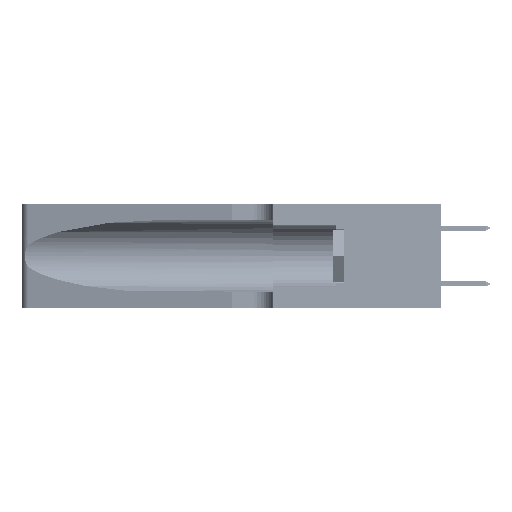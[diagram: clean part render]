
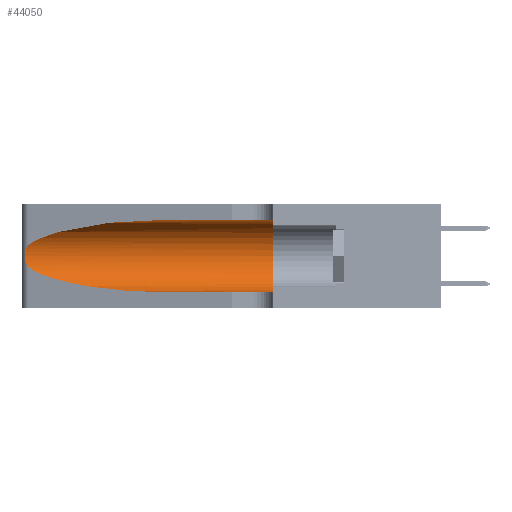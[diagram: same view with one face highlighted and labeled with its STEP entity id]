
A CAD part, left-side view. The second image highlights one B-rep face of the part: STEP entity #44050.
In plain terms, the highlighted cylindrical face has radius 3.308 mm (diameter 6.617 mm), a partial arc.
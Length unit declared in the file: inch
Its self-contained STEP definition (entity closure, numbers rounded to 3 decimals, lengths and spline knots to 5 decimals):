
#435 = EDGE_CURVE ( 'NONE', #28097, #11535, #31660, .T. ) ;
#770 =( BOUNDED_CURVE ( )  B_SPLINE_CURVE ( 3, ( #2376, #9634, #16891, #41782 ),
 .UNSPECIFIED., .F., .F. ) 
 B_SPLINE_CURVE_WITH_KNOTS ( ( 4, 4 ),
 ( 1.5708, 2.84003 ),
 .UNSPECIFIED. ) 
 CURVE ( )  GEOMETRIC_REPRESENTATION_ITEM ( )  RATIONAL_B_SPLINE_CURVE ( ( 1., 0.87, 0.87, 1. ) ) 
 REPRESENTATION_ITEM ( '' )  );
#802 = DIRECTION ( 'NONE',  ( 0., 0., -1. ) ) ;
#2350 = CARTESIAN_POINT ( 'NONE',  ( 0.1305, 0.72297, 0.05475 ) ) ;
#2376 = CARTESIAN_POINT ( 'NONE',  ( 0.1305, 0.72297, 0.31525 ) ) ;
#3324 = ORIENTED_EDGE ( 'NONE', *, *, #16526, .F. ) ;
#3594 = CARTESIAN_POINT ( 'NONE',  ( 0.25639, 1.23186, 0.15144 ) ) ;
#6356 = CIRCLE ( 'NONE', #20125, 0.13025 ) ;
#7041 = CARTESIAN_POINT ( 'NONE',  ( 0.25555, 1.22994, 0.2215 ) ) ;
#7211 = CARTESIAN_POINT ( 'NONE',  ( 0.25487, 1.22718, 0.14631 ) ) ;
#7308 = EDGE_CURVE ( 'NONE', #9059, #24847, #37540, .T. ) ;
#8315 = CARTESIAN_POINT ( 'NONE',  ( 0.1305, 1.61858, 0.31525 ) ) ;
#8981 = VECTOR ( 'NONE', #22876, 39.37008 ) ;
#9059 = VERTEX_POINT ( 'NONE', #37400 ) ;
#9634 = CARTESIAN_POINT ( 'NONE',  ( 0.18966, 0.96281, 0.31525 ) ) ;
#10125 = AXIS2_PLACEMENT_3D ( 'NONE', #22480, #15165, #802 ) ;
#10717 = CARTESIAN_POINT ( 'NONE',  ( 0.25639, 1.23184, 0.21858 ) ) ;
#10972 = CARTESIAN_POINT ( 'NONE',  ( 0.2373, 1.15595, 0.08982 ) ) ;
#11535 = VERTEX_POINT ( 'NONE', #2350 ) ;
#13559 = CARTESIAN_POINT ( 'NONE',  ( 0.25487, 1.22718, 0.22369 ) ) ;
#13665 = EDGE_CURVE ( 'NONE', #30911, #28097, #21604, .T. ) ;
#14311 = CARTESIAN_POINT ( 'NONE',  ( 0.25854, 1.2359, 0.20912 ) ) ;
#15165 = DIRECTION ( 'NONE',  ( 0., -1., 0. ) ) ;
#15543 = CARTESIAN_POINT ( 'NONE',  ( 0.25487, 1.22718, 0.14631 ) ) ;
#16480 = CARTESIAN_POINT ( 'NONE',  ( 0.1305, 1.61858, 0.05475 ) ) ;
#16526 = EDGE_CURVE ( 'NONE', #24847, #32883, #6356, .T. ) ;
#16591 = CARTESIAN_POINT ( 'NONE',  ( 0.1305, 0.35, 0.31525 ) ) ;
#16891 = CARTESIAN_POINT ( 'NONE',  ( 0.2373, 1.15595, 0.28018 ) ) ;
#17970 = CARTESIAN_POINT ( 'NONE',  ( 0.26075, 1.23896, 0.19203 ) ) ;
#18861 = EDGE_CURVE ( 'NONE', #9059, #30911, #770, .T. ) ;
#19762 = CARTESIAN_POINT ( 'NONE',  ( 0.25856, 1.23593, 0.16098 ) ) ;
#19768 = DIRECTION ( 'NONE',  ( 0., 1., 0. ) ) ;
#20125 = AXIS2_PLACEMENT_3D ( 'NONE', #41024, #19768, #44546 ) ;
#20153 = DIRECTION ( 'NONE',  ( 0., -1., 0. ) ) ;
#20657 = VECTOR ( 'NONE', #20153, 39.37008 ) ;
#21604 = B_SPLINE_CURVE_WITH_KNOTS ( 'NONE', 3,
 ( #39135, #7041, #10717, #35744, #14311, #39286, #17970, #42828, #21638, #19762, #25254, #3594, #28826, #7211 ),
 .UNSPECIFIED., .F., .F.,
 ( 4, 2, 2, 2, 2, 2, 4 ),
 ( 0., 0.00027, 0.00053, 0.00107, 0.0016, 0.00187, 0.00214 ),
 .UNSPECIFIED. ) ;
#21638 = CARTESIAN_POINT ( 'NONE',  ( 0.26017, 1.23833, 0.17102 ) ) ;
#21849 = CARTESIAN_POINT ( 'NONE',  ( 0.1305, 0.35, 0.05475 ) ) ;
#21883 = EDGE_CURVE ( 'NONE', #11535, #32883, #38412, .T. ) ;
#22182 = CYLINDRICAL_SURFACE ( 'NONE', #10125, 0.13025 ) ;
#22480 = CARTESIAN_POINT ( 'NONE',  ( 0.1305, 1.61858, 0.185 ) ) ;
#22876 = DIRECTION ( 'NONE',  ( 0., -1., 0. ) ) ;
#24847 = VERTEX_POINT ( 'NONE', #16591 ) ;
#25254 = CARTESIAN_POINT ( 'NONE',  ( 0.25789, 1.23486, 0.15765 ) ) ;
#25903 = ORIENTED_EDGE ( 'NONE', *, *, #18861, .T. ) ;
#27582 = ORIENTED_EDGE ( 'NONE', *, *, #21883, .T. ) ;
#28097 = VERTEX_POINT ( 'NONE', #15543 ) ;
#28826 = CARTESIAN_POINT ( 'NONE',  ( 0.25555, 1.22993, 0.14849 ) ) ;
#30911 = VERTEX_POINT ( 'NONE', #13559 ) ;
#31660 =( BOUNDED_CURVE ( )  B_SPLINE_CURVE ( 3, ( #35997, #10972, #32488, #39542 ),
 .UNSPECIFIED., .F., .F. ) 
 B_SPLINE_CURVE_WITH_KNOTS ( ( 4, 4 ),
 ( 3.44316, 4.71239 ),
 .UNSPECIFIED. ) 
 CURVE ( )  GEOMETRIC_REPRESENTATION_ITEM ( )  RATIONAL_B_SPLINE_CURVE ( ( 1., 0.87, 0.87, 1. ) ) 
 REPRESENTATION_ITEM ( '' )  );
#32488 = CARTESIAN_POINT ( 'NONE',  ( 0.18966, 0.96281, 0.05475 ) ) ;
#32883 = VERTEX_POINT ( 'NONE', #21849 ) ;
#32924 = EDGE_LOOP ( 'NONE', ( #25903, #43014, #35848, #27582, #3324, #34243 ) ) ;
#34243 = ORIENTED_EDGE ( 'NONE', *, *, #7308, .F. ) ;
#35744 = CARTESIAN_POINT ( 'NONE',  ( 0.25787, 1.23484, 0.2124 ) ) ;
#35848 = ORIENTED_EDGE ( 'NONE', *, *, #435, .T. ) ;
#35997 = CARTESIAN_POINT ( 'NONE',  ( 0.25487, 1.22718, 0.14631 ) ) ;
#37400 = CARTESIAN_POINT ( 'NONE',  ( 0.1305, 0.72297, 0.31525 ) ) ;
#37540 = LINE ( 'NONE', #8315, #8981 ) ;
#38412 = LINE ( 'NONE', #16480, #20657 ) ;
#39135 = CARTESIAN_POINT ( 'NONE',  ( 0.25487, 1.22718, 0.22369 ) ) ;
#39286 = CARTESIAN_POINT ( 'NONE',  ( 0.26018, 1.23835, 0.19895 ) ) ;
#39542 = CARTESIAN_POINT ( 'NONE',  ( 0.1305, 0.72297, 0.05475 ) ) ;
#41016 = FACE_OUTER_BOUND ( 'NONE', #32924, .T. ) ;
#41024 = CARTESIAN_POINT ( 'NONE',  ( 0.1305, 0.35, 0.185 ) ) ;
#41782 = CARTESIAN_POINT ( 'NONE',  ( 0.25487, 1.22718, 0.22369 ) ) ;
#42828 = CARTESIAN_POINT ( 'NONE',  ( 0.26075, 1.23896, 0.178 ) ) ;
#43014 = ORIENTED_EDGE ( 'NONE', *, *, #13665, .T. ) ;
#44050 = ADVANCED_FACE ( 'NONE', ( #41016 ), #22182, .F. ) ;
#44546 = DIRECTION ( 'NONE',  ( 0., 0., 1. ) ) ;
